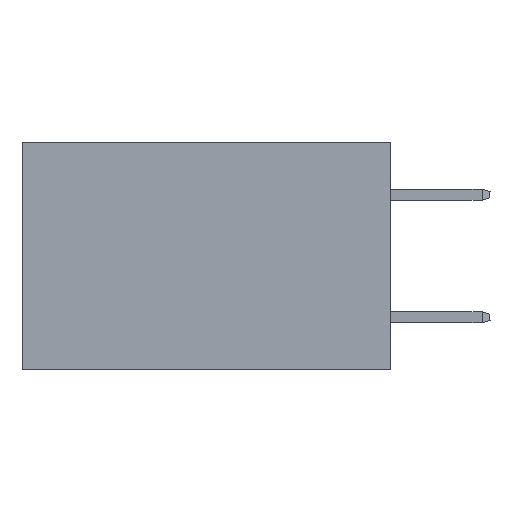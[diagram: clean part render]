
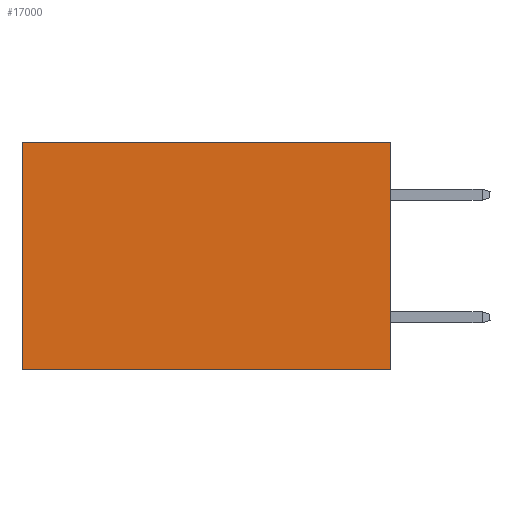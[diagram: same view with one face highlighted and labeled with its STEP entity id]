
A CAD part, left-side view. The second image highlights one B-rep face of the part: STEP entity #17000.
In plain terms, the highlighted planar face has unit normal (-1, 0, 0).
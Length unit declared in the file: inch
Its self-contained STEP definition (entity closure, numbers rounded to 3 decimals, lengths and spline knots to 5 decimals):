
#963 = EDGE_CURVE ( 'NONE', #19768, #26582, #19363, .T. ) ;
#2113 = CARTESIAN_POINT ( 'NONE',  ( 0.2875, 0., 0. ) ) ;
#2131 = FACE_OUTER_BOUND ( 'NONE', #12358, .T. ) ;
#2509 = ORIENTED_EDGE ( 'NONE', *, *, #963, .F. ) ;
#3008 = CARTESIAN_POINT ( 'NONE',  ( 0.2875, 0.6, 0. ) ) ;
#3588 = DIRECTION ( 'NONE',  ( 0., 0., -1. ) ) ;
#3974 = CARTESIAN_POINT ( 'NONE',  ( 0.2875, 0., 0. ) ) ;
#4647 = VERTEX_POINT ( 'NONE', #24265 ) ;
#5000 = EDGE_CURVE ( 'NONE', #20653, #4647, #23154, .T. ) ;
#5492 = DIRECTION ( 'NONE',  ( 0., 1., 0. ) ) ;
#5515 = LINE ( 'NONE', #24190, #14033 ) ;
#9033 = CARTESIAN_POINT ( 'NONE',  ( 0.2875, 0., -0.37 ) ) ;
#9367 = ORIENTED_EDGE ( 'NONE', *, *, #10065, .F. ) ;
#10065 = EDGE_CURVE ( 'NONE', #26582, #4647, #5515, .T. ) ;
#10082 = CARTESIAN_POINT ( 'NONE',  ( 0.2875, 0., 0. ) ) ;
#11695 = DIRECTION ( 'NONE',  ( 0., 0., -1. ) ) ;
#12358 = EDGE_LOOP ( 'NONE', ( #18643, #9367, #2509, #20133 ) ) ;
#12879 = EDGE_CURVE ( 'NONE', #19768, #20653, #14211, .T. ) ;
#14033 = VECTOR ( 'NONE', #5492, 39.37008 ) ;
#14211 = LINE ( 'NONE', #2113, #23862 ) ;
#14722 = DIRECTION ( 'NONE',  ( 0., 1., 0. ) ) ;
#16614 = PLANE ( 'NONE',  #17683 ) ;
#17000 = ADVANCED_FACE ( 'NONE', ( #2131 ), #16614, .F. ) ;
#17080 = VECTOR ( 'NONE', #3588, 39.37008 ) ;
#17683 = AXIS2_PLACEMENT_3D ( 'NONE', #21874, #17924, #11695 ) ;
#17924 = DIRECTION ( 'NONE',  ( 1., 0., 0. ) ) ;
#18643 = ORIENTED_EDGE ( 'NONE', *, *, #5000, .T. ) ;
#19072 = DIRECTION ( 'NONE',  ( 0., 0., -1. ) ) ;
#19363 = LINE ( 'NONE', #10082, #17080 ) ;
#19768 = VERTEX_POINT ( 'NONE', #3974 ) ;
#20133 = ORIENTED_EDGE ( 'NONE', *, *, #12879, .T. ) ;
#20653 = VERTEX_POINT ( 'NONE', #3008 ) ;
#21874 = CARTESIAN_POINT ( 'NONE',  ( 0.2875, 0., 0. ) ) ;
#22230 = VECTOR ( 'NONE', #19072, 39.37008 ) ;
#23154 = LINE ( 'NONE', #25221, #22230 ) ;
#23862 = VECTOR ( 'NONE', #14722, 39.37008 ) ;
#24190 = CARTESIAN_POINT ( 'NONE',  ( 0.2875, 0., -0.37 ) ) ;
#24265 = CARTESIAN_POINT ( 'NONE',  ( 0.2875, 0.6, -0.37 ) ) ;
#25221 = CARTESIAN_POINT ( 'NONE',  ( 0.2875, 0.6, 0. ) ) ;
#26582 = VERTEX_POINT ( 'NONE', #9033 ) ;
